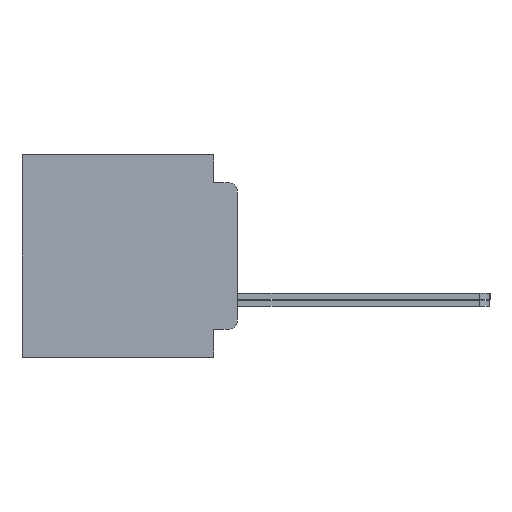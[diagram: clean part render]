
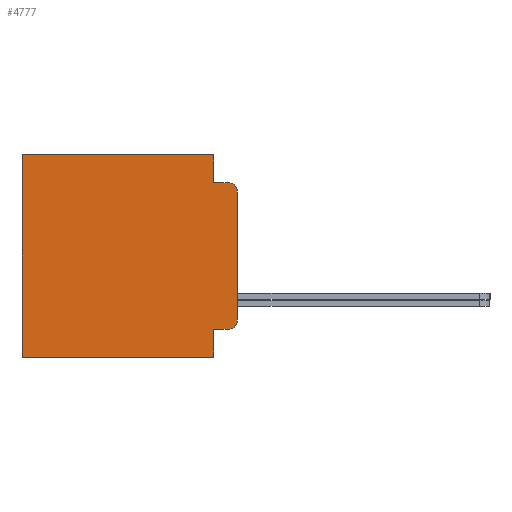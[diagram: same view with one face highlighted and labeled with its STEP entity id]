
A CAD part, left-side view. The second image highlights one B-rep face of the part: STEP entity #4777.
In plain terms, the highlighted planar face has unit normal (-1, 0, 0).
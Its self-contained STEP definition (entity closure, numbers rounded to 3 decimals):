
#74 = VERTEX_POINT ( 'NONE', #21217 ) ;
#286 = CIRCLE ( 'NONE', #17214, 0.508 ) ;
#554 = CARTESIAN_POINT ( 'NONE',  ( -67.462, 1.295, 5.486 ) ) ;
#1014 = CARTESIAN_POINT ( 'NONE',  ( -67.462, 0., -5.486 ) ) ;
#1039 = AXIS2_PLACEMENT_3D ( 'NONE', #13889, #7542, #24493 ) ;
#1462 = VERTEX_POINT ( 'NONE', #24405 ) ;
#1631 = CARTESIAN_POINT ( 'NONE',  ( -67.462, 0.508, -3.467 ) ) ;
#1932 = VECTOR ( 'NONE', #23905, 1000. ) ;
#2576 = EDGE_CURVE ( 'NONE', #21528, #11171, #6488, .T. ) ;
#2752 = VECTOR ( 'NONE', #13292, 1000. ) ;
#2839 = ORIENTED_EDGE ( 'NONE', *, *, #12622, .F. ) ;
#2875 = DIRECTION ( 'NONE',  ( 0., 0., -1. ) ) ;
#3165 = VERTEX_POINT ( 'NONE', #9426 ) ;
#3592 = CIRCLE ( 'NONE', #1039, 0.508 ) ;
#4413 = VECTOR ( 'NONE', #9358, 1000. ) ;
#4632 = CARTESIAN_POINT ( 'NONE',  ( -67.462, 0., -3.467 ) ) ;
#4777 = ADVANCED_FACE ( 'NONE', ( #5435 ), #17737, .F. ) ;
#5435 = FACE_OUTER_BOUND ( 'NONE', #9864, .T. ) ;
#5600 = EDGE_CURVE ( 'NONE', #26199, #11171, #17507, .T. ) ;
#5861 = DIRECTION ( 'NONE',  ( 0., 0., -1. ) ) ;
#6488 = LINE ( 'NONE', #20013, #19653 ) ;
#6752 = EDGE_CURVE ( 'NONE', #26288, #26199, #9924, .T. ) ;
#7002 = ORIENTED_EDGE ( 'NONE', *, *, #26954, .F. ) ;
#7093 = CARTESIAN_POINT ( 'NONE',  ( -67.462, 0., -5.486 ) ) ;
#7415 = ORIENTED_EDGE ( 'NONE', *, *, #2576, .F. ) ;
#7542 = DIRECTION ( 'NONE',  ( -1., 0., 0. ) ) ;
#8747 = CARTESIAN_POINT ( 'NONE',  ( -67.462, 11.684, 5.486 ) ) ;
#8771 = CARTESIAN_POINT ( 'NONE',  ( -67.462, 1.295, -5.486 ) ) ;
#9346 = LINE ( 'NONE', #13503, #4413 ) ;
#9358 = DIRECTION ( 'NONE',  ( 0., 0., -1. ) ) ;
#9426 = CARTESIAN_POINT ( 'NONE',  ( -67.462, 0.508, 3.975 ) ) ;
#9864 = EDGE_LOOP ( 'NONE', ( #14730, #25100, #16863, #21859, #2839, #7002, #24073, #17493, #7415, #11833 ) ) ;
#9924 = LINE ( 'NONE', #20861, #12545 ) ;
#10180 = EDGE_CURVE ( 'NONE', #1462, #19758, #10386, .T. ) ;
#10386 = LINE ( 'NONE', #7093, #26541 ) ;
#10605 = LINE ( 'NONE', #22798, #25423 ) ;
#11049 = VERTEX_POINT ( 'NONE', #14149 ) ;
#11171 = VERTEX_POINT ( 'NONE', #13745 ) ;
#11351 = DIRECTION ( 'NONE',  ( 0., 0., -1. ) ) ;
#11833 = ORIENTED_EDGE ( 'NONE', *, *, #15714, .F. ) ;
#12545 = VECTOR ( 'NONE', #14623, 1000. ) ;
#12622 = EDGE_CURVE ( 'NONE', #20717, #3165, #10605, .T. ) ;
#13292 = DIRECTION ( 'NONE',  ( 0., 0., -1. ) ) ;
#13503 = CARTESIAN_POINT ( 'NONE',  ( -67.462, 1.295, 0. ) ) ;
#13745 = CARTESIAN_POINT ( 'NONE',  ( -67.462, 11.684, -5.486 ) ) ;
#13889 = CARTESIAN_POINT ( 'NONE',  ( -67.462, 0.508, 3.467 ) ) ;
#14079 = DIRECTION ( 'NONE',  ( 0., 0., -1. ) ) ;
#14149 = CARTESIAN_POINT ( 'NONE',  ( -67.462, 0.508, -3.975 ) ) ;
#14623 = DIRECTION ( 'NONE',  ( 0., 1., 0. ) ) ;
#14730 = ORIENTED_EDGE ( 'NONE', *, *, #24069, .T. ) ;
#15695 = VECTOR ( 'NONE', #14079, 1000. ) ;
#15714 = EDGE_CURVE ( 'NONE', #74, #21528, #21629, .T. ) ;
#16863 = ORIENTED_EDGE ( 'NONE', *, *, #10180, .F. ) ;
#17008 = LINE ( 'NONE', #17602, #1932 ) ;
#17214 = AXIS2_PLACEMENT_3D ( 'NONE', #1631, #18166, #5861 ) ;
#17493 = ORIENTED_EDGE ( 'NONE', *, *, #5600, .T. ) ;
#17507 = LINE ( 'NONE', #23609, #2752 ) ;
#17602 = CARTESIAN_POINT ( 'NONE',  ( -67.462, 1.295, -3.975 ) ) ;
#17737 = PLANE ( 'NONE',  #26999 ) ;
#18166 = DIRECTION ( 'NONE',  ( -1., 0., 0. ) ) ;
#19653 = VECTOR ( 'NONE', #24028, 1000. ) ;
#19758 = VERTEX_POINT ( 'NONE', #4632 ) ;
#19852 = DIRECTION ( 'NONE',  ( 1., 0., 0. ) ) ;
#20013 = CARTESIAN_POINT ( 'NONE',  ( -67.462, 0., -5.486 ) ) ;
#20492 = CARTESIAN_POINT ( 'NONE',  ( -67.462, 1.295, 3.975 ) ) ;
#20643 = DIRECTION ( 'NONE',  ( 0., -1., 0. ) ) ;
#20717 = VERTEX_POINT ( 'NONE', #20492 ) ;
#20861 = CARTESIAN_POINT ( 'NONE',  ( -67.462, 0., 5.486 ) ) ;
#21217 = CARTESIAN_POINT ( 'NONE',  ( -67.462, 1.295, -3.975 ) ) ;
#21307 = EDGE_CURVE ( 'NONE', #11049, #19758, #286, .T. ) ;
#21528 = VERTEX_POINT ( 'NONE', #8771 ) ;
#21629 = LINE ( 'NONE', #22449, #15695 ) ;
#21859 = ORIENTED_EDGE ( 'NONE', *, *, #22491, .T. ) ;
#22449 = CARTESIAN_POINT ( 'NONE',  ( -67.462, 1.295, 0. ) ) ;
#22491 = EDGE_CURVE ( 'NONE', #1462, #3165, #3592, .T. ) ;
#22798 = CARTESIAN_POINT ( 'NONE',  ( -67.462, 1.295, 3.975 ) ) ;
#23609 = CARTESIAN_POINT ( 'NONE',  ( -67.462, 11.684, -5.486 ) ) ;
#23905 = DIRECTION ( 'NONE',  ( 0., -1., 0. ) ) ;
#24028 = DIRECTION ( 'NONE',  ( 0., 1., 0. ) ) ;
#24069 = EDGE_CURVE ( 'NONE', #74, #11049, #17008, .T. ) ;
#24073 = ORIENTED_EDGE ( 'NONE', *, *, #6752, .T. ) ;
#24405 = CARTESIAN_POINT ( 'NONE',  ( -67.462, 0., 3.467 ) ) ;
#24493 = DIRECTION ( 'NONE',  ( 0., 0., -1. ) ) ;
#25100 = ORIENTED_EDGE ( 'NONE', *, *, #21307, .T. ) ;
#25423 = VECTOR ( 'NONE', #20643, 1000. ) ;
#26199 = VERTEX_POINT ( 'NONE', #8747 ) ;
#26288 = VERTEX_POINT ( 'NONE', #554 ) ;
#26541 = VECTOR ( 'NONE', #11351, 1000. ) ;
#26954 = EDGE_CURVE ( 'NONE', #26288, #20717, #9346, .T. ) ;
#26999 = AXIS2_PLACEMENT_3D ( 'NONE', #1014, #19852, #2875 ) ;
